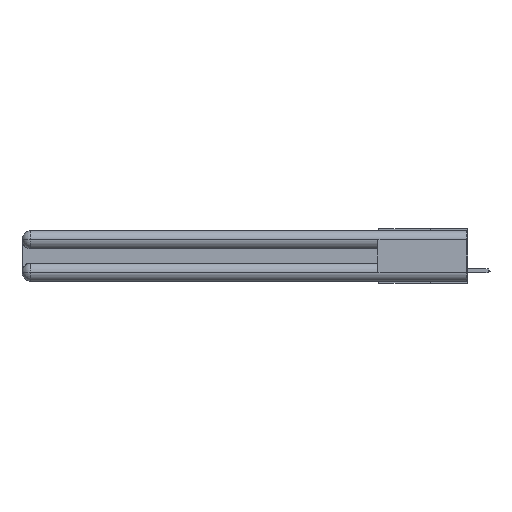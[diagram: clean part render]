
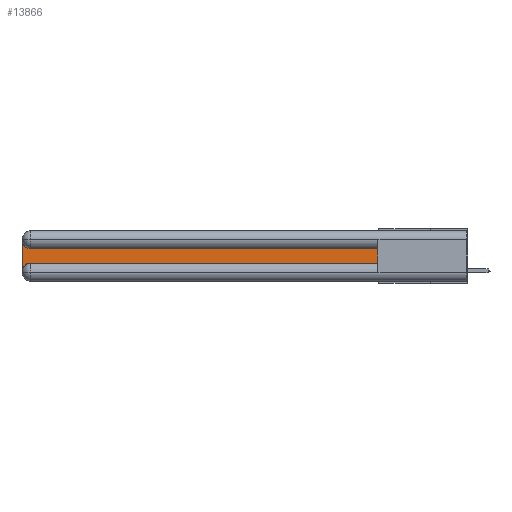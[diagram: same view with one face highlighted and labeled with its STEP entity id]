
A CAD part, left-side view. The second image highlights one B-rep face of the part: STEP entity #13866.
In plain terms, the highlighted planar face has unit normal (-1, 0, 0).
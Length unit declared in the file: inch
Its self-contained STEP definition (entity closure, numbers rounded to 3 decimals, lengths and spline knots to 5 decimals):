
#1062 = VECTOR ( 'NONE', #6130, 39.37008 ) ;
#1177 = ORIENTED_EDGE ( 'NONE', *, *, #20201, .T. ) ;
#1456 = LINE ( 'NONE', #16898, #27916 ) ;
#1763 = DIRECTION ( 'NONE',  ( 1., 0., 0. ) ) ;
#2161 = CARTESIAN_POINT ( 'NONE',  ( 0.075, 2.94, -0.1225 ) ) ;
#2825 = VERTEX_POINT ( 'NONE', #31170 ) ;
#3762 = DIRECTION ( 'NONE',  ( 0., -1., 0. ) ) ;
#3898 = EDGE_CURVE ( 'NONE', #2825, #22428, #32549, .T. ) ;
#4295 = EDGE_LOOP ( 'NONE', ( #15921, #18500, #23643, #11525, #20830, #1177 ) ) ;
#4364 = AXIS2_PLACEMENT_3D ( 'NONE', #7416, #28051, #12462 ) ;
#4614 = FACE_OUTER_BOUND ( 'NONE', #4295, .T. ) ;
#5778 = EDGE_CURVE ( 'NONE', #20291, #2825, #15152, .T. ) ;
#5923 = EDGE_CURVE ( 'NONE', #22428, #16101, #1456, .T. ) ;
#6130 = DIRECTION ( 'NONE',  ( 0., 0., -1. ) ) ;
#6320 = AXIS2_PLACEMENT_3D ( 'NONE', #12098, #30343, #14795 ) ;
#7416 = CARTESIAN_POINT ( 'NONE',  ( 0.075, 3., -0.1225 ) ) ;
#8538 = CARTESIAN_POINT ( 'NONE',  ( 0.075, 0.6, -0.2175 ) ) ;
#8642 = CARTESIAN_POINT ( 'NONE',  ( 0.075, 2.94, -0.2175 ) ) ;
#11525 = ORIENTED_EDGE ( 'NONE', *, *, #3898, .T. ) ;
#12098 = CARTESIAN_POINT ( 'NONE',  ( 0.075, 2.94, -0.2775 ) ) ;
#12462 = DIRECTION ( 'NONE',  ( 0., 0., -1. ) ) ;
#12846 = CIRCLE ( 'NONE', #31912, 0.06 ) ;
#13866 = ADVANCED_FACE ( 'NONE', ( #4614 ), #15388, .F. ) ;
#14544 = VECTOR ( 'NONE', #17464, 39.37008 ) ;
#14795 = DIRECTION ( 'NONE',  ( 0., 0., -1. ) ) ;
#15152 = LINE ( 'NONE', #26327, #1062 ) ;
#15388 = PLANE ( 'NONE',  #4364 ) ;
#15868 = VERTEX_POINT ( 'NONE', #2161 ) ;
#15921 = ORIENTED_EDGE ( 'NONE', *, *, #20741, .T. ) ;
#16101 = VERTEX_POINT ( 'NONE', #8538 ) ;
#16898 = CARTESIAN_POINT ( 'NONE',  ( 0.075, 0.6, -0.2175 ) ) ;
#17147 = CARTESIAN_POINT ( 'NONE',  ( 0.075, 2.94, -0.0625 ) ) ;
#17464 = DIRECTION ( 'NONE',  ( 0., 1., 0. ) ) ;
#18500 = ORIENTED_EDGE ( 'NONE', *, *, #30552, .T. ) ;
#20201 = EDGE_CURVE ( 'NONE', #16101, #21560, #32275, .T. ) ;
#20291 = VERTEX_POINT ( 'NONE', #30857 ) ;
#20741 = EDGE_CURVE ( 'NONE', #21560, #15868, #21362, .T. ) ;
#20830 = ORIENTED_EDGE ( 'NONE', *, *, #5923, .T. ) ;
#21362 = LINE ( 'NONE', #30120, #14544 ) ;
#21560 = VERTEX_POINT ( 'NONE', #25523 ) ;
#22428 = VERTEX_POINT ( 'NONE', #8642 ) ;
#23643 = ORIENTED_EDGE ( 'NONE', *, *, #5778, .T. ) ;
#24812 = DIRECTION ( 'NONE',  ( 0., 0., 1. ) ) ;
#25523 = CARTESIAN_POINT ( 'NONE',  ( 0.075, 0.6, -0.1225 ) ) ;
#26327 = CARTESIAN_POINT ( 'NONE',  ( 0.075, 3., -0.2175 ) ) ;
#27273 = CARTESIAN_POINT ( 'NONE',  ( 0.075, 0.6, -0.2175 ) ) ;
#27916 = VECTOR ( 'NONE', #3762, 39.37008 ) ;
#28051 = DIRECTION ( 'NONE',  ( 1., 0., 0. ) ) ;
#29816 = VECTOR ( 'NONE', #24812, 39.37008 ) ;
#30120 = CARTESIAN_POINT ( 'NONE',  ( 0.075, 0.6, -0.1225 ) ) ;
#30343 = DIRECTION ( 'NONE',  ( 1., 0., 0. ) ) ;
#30552 = EDGE_CURVE ( 'NONE', #15868, #20291, #12846, .T. ) ;
#30857 = CARTESIAN_POINT ( 'NONE',  ( 0.075, 3., -0.0625 ) ) ;
#31170 = CARTESIAN_POINT ( 'NONE',  ( 0.075, 3., -0.2775 ) ) ;
#31912 = AXIS2_PLACEMENT_3D ( 'NONE', #17147, #1763, #32080 ) ;
#32080 = DIRECTION ( 'NONE',  ( 0., 0., -1. ) ) ;
#32275 = LINE ( 'NONE', #27273, #29816 ) ;
#32549 = CIRCLE ( 'NONE', #6320, 0.06 ) ;
